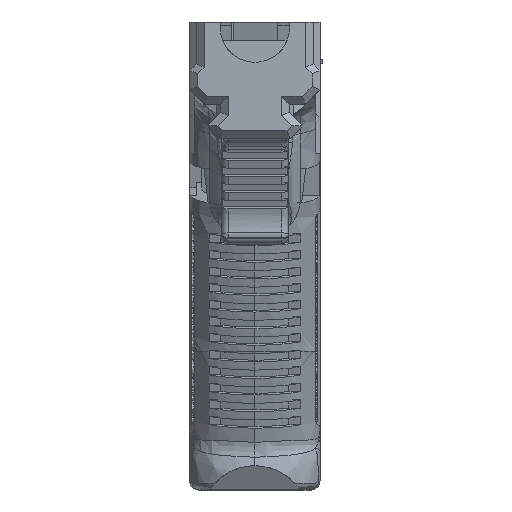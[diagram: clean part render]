
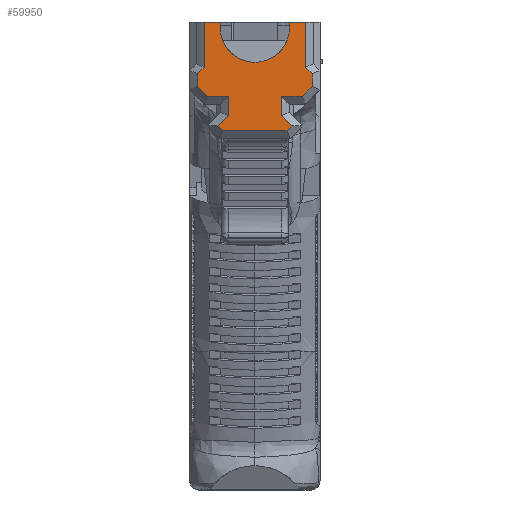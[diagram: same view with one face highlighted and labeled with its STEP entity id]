
A CAD part, left-side view. The second image highlights one B-rep face of the part: STEP entity #59950.
In plain terms, the highlighted planar face has unit normal (-1, 0, 0).
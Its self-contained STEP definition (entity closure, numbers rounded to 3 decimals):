
#7520=PLANE('',#61345);
#7623=LINE('',#68131,#11348);
#7689=LINE('',#70585,#11414);
#10973=LINE('',#139716,#14698);
#10977=LINE('',#139723,#14702);
#10980=LINE('',#139728,#14705);
#10982=LINE('',#139732,#14707);
#10984=LINE('',#139736,#14709);
#10986=LINE('',#139741,#14711);
#10997=LINE('',#139763,#14722);
#11000=LINE('',#139768,#14725);
#11002=LINE('',#139773,#14727);
#11014=LINE('',#139798,#14739);
#11016=LINE('',#139802,#14741);
#11018=LINE('',#139806,#14743);
#11020=LINE('',#139810,#14745);
#11022=LINE('',#139814,#14747);
#11025=LINE('',#139819,#14750);
#11239=LINE('',#142619,#14964);
#11241=LINE('',#142623,#14966);
#11242=LINE('',#142624,#14967);
#11243=LINE('',#142625,#14968);
#11348=VECTOR('',#61560,10.);
#11414=VECTOR('',#61656,10.);
#14698=VECTOR('',#67150,10.);
#14702=VECTOR('',#67156,10.);
#14705=VECTOR('',#67161,10.);
#14707=VECTOR('',#67165,10.);
#14709=VECTOR('',#67169,10.);
#14711=VECTOR('',#67173,10.);
#14722=VECTOR('',#67196,10.);
#14725=VECTOR('',#67201,10.);
#14727=VECTOR('',#67205,10.);
#14739=VECTOR('',#67229,10.);
#14741=VECTOR('',#67233,10.);
#14743=VECTOR('',#67237,10.);
#14745=VECTOR('',#67241,10.);
#14747=VECTOR('',#67245,10.);
#14750=VECTOR('',#67250,10.);
#14964=VECTOR('',#67768,10.);
#14966=VECTOR('',#67774,10.);
#14967=VECTOR('',#67775,10.);
#14968=VECTOR('',#67776,10.);
#18471=FACE_OUTER_BOUND('',#22299,.T.);
#22299=EDGE_LOOP('',(#56180,#56181,#56182,#56183,#56184,#56185,#56186,#56187,
#56188,#56189,#56190,#56191,#56192,#56193,#56194,#56195,#56196,#56197,#56198,
#56199,#56200,#56201));
#22546=CIRCLE('',#61247,7.765);
#23861=VERTEX_POINT('',#68128);
#23862=VERTEX_POINT('',#68130);
#24009=VERTEX_POINT('',#70582);
#24010=VERTEX_POINT('',#70584);
#29482=VERTEX_POINT('',#139713);
#29483=VERTEX_POINT('',#139715);
#29485=VERTEX_POINT('',#139721);
#29486=VERTEX_POINT('',#139726);
#29487=VERTEX_POINT('',#139730);
#29488=VERTEX_POINT('',#139734);
#29489=VERTEX_POINT('',#139738);
#29495=VERTEX_POINT('',#139762);
#29496=VERTEX_POINT('',#139766);
#29497=VERTEX_POINT('',#139770);
#29505=VERTEX_POINT('',#139797);
#29506=VERTEX_POINT('',#139801);
#29507=VERTEX_POINT('',#139805);
#29508=VERTEX_POINT('',#139809);
#29509=VERTEX_POINT('',#139813);
#29510=VERTEX_POINT('',#139818);
#29555=VERTEX_POINT('',#141368);
#29556=VERTEX_POINT('',#141370);
#29803=EDGE_CURVE('',#23862,#23861,#7623,.T.);
#29962=EDGE_CURVE('',#24010,#24009,#7689,.T.);
#38209=EDGE_CURVE('',#29482,#29483,#10973,.T.);
#38213=EDGE_CURVE('',#29485,#29482,#10977,.T.);
#38216=EDGE_CURVE('',#29486,#29485,#10980,.T.);
#38218=EDGE_CURVE('',#29487,#29486,#10982,.T.);
#38220=EDGE_CURVE('',#29488,#29487,#10984,.T.);
#38222=EDGE_CURVE('',#29489,#29488,#10986,.T.);
#38233=EDGE_CURVE('',#29495,#29489,#10997,.T.);
#38236=EDGE_CURVE('',#29496,#29495,#11000,.T.);
#38238=EDGE_CURVE('',#29497,#29496,#11002,.T.);
#38250=EDGE_CURVE('',#29505,#29497,#11014,.T.);
#38252=EDGE_CURVE('',#29506,#29505,#11016,.T.);
#38254=EDGE_CURVE('',#29507,#29506,#11018,.T.);
#38256=EDGE_CURVE('',#29508,#29507,#11020,.T.);
#38258=EDGE_CURVE('',#29509,#29508,#11022,.T.);
#38261=EDGE_CURVE('',#29510,#29509,#11025,.T.);
#38364=EDGE_CURVE('',#29556,#29555,#22546,.T.);
#38606=EDGE_CURVE('',#29483,#24009,#11239,.T.);
#38608=EDGE_CURVE('',#23861,#29556,#11241,.T.);
#38609=EDGE_CURVE('',#29555,#24010,#11242,.T.);
#38610=EDGE_CURVE('',#23862,#29510,#11243,.T.);
#56180=ORIENTED_EDGE('',*,*,#29803,.T.);
#56181=ORIENTED_EDGE('',*,*,#38608,.T.);
#56182=ORIENTED_EDGE('',*,*,#38364,.T.);
#56183=ORIENTED_EDGE('',*,*,#38609,.T.);
#56184=ORIENTED_EDGE('',*,*,#29962,.T.);
#56185=ORIENTED_EDGE('',*,*,#38606,.F.);
#56186=ORIENTED_EDGE('',*,*,#38209,.F.);
#56187=ORIENTED_EDGE('',*,*,#38213,.F.);
#56188=ORIENTED_EDGE('',*,*,#38216,.F.);
#56189=ORIENTED_EDGE('',*,*,#38218,.F.);
#56190=ORIENTED_EDGE('',*,*,#38220,.F.);
#56191=ORIENTED_EDGE('',*,*,#38222,.F.);
#56192=ORIENTED_EDGE('',*,*,#38233,.F.);
#56193=ORIENTED_EDGE('',*,*,#38236,.F.);
#56194=ORIENTED_EDGE('',*,*,#38238,.F.);
#56195=ORIENTED_EDGE('',*,*,#38250,.F.);
#56196=ORIENTED_EDGE('',*,*,#38252,.F.);
#56197=ORIENTED_EDGE('',*,*,#38254,.F.);
#56198=ORIENTED_EDGE('',*,*,#38256,.F.);
#56199=ORIENTED_EDGE('',*,*,#38258,.F.);
#56200=ORIENTED_EDGE('',*,*,#38261,.F.);
#56201=ORIENTED_EDGE('',*,*,#38610,.F.);
#59950=ADVANCED_FACE('',(#18471),#7520,.F.);
#61247=AXIS2_PLACEMENT_3D('',#141371,#67410,#67411);
#61345=AXIS2_PLACEMENT_3D('',#142622,#67772,#67773);
#61560=DIRECTION('',(0.,1.,0.));
#61656=DIRECTION('',(0.,1.,0.));
#67150=DIRECTION('',(0.,-0.707,0.707));
#67156=DIRECTION('',(0.,0.,1.));
#67161=DIRECTION('',(0.,0.707,0.707));
#67165=DIRECTION('',(0.,1.,0.));
#67169=DIRECTION('',(0.,0.,1.));
#67173=DIRECTION('',(0.,-0.707,0.707));
#67196=DIRECTION('',(0.,0.707,0.707));
#67201=DIRECTION('',(0.,1.,0.));
#67205=DIRECTION('',(0.,0.707,-0.707));
#67229=DIRECTION('',(0.,-0.707,-0.707));
#67233=DIRECTION('',(0.,0.,-1.));
#67237=DIRECTION('',(0.,1.,0.));
#67241=DIRECTION('',(0.,0.707,-0.707));
#67245=DIRECTION('',(0.,0.,-1.));
#67250=DIRECTION('',(0.,-0.707,-0.707));
#67410=DIRECTION('center_axis',(1.,0.,0.));
#67411=DIRECTION('ref_axis',(0.,0.,
-1.));
#67768=DIRECTION('',(0.,0.,1.));
#67772=DIRECTION('center_axis',(1.,0.,0.));
#67773=DIRECTION('ref_axis',(0.,0.,
1.));
#67774=DIRECTION('',(0.,0.,-1.));
#67775=DIRECTION('',(0.,0.,1.));
#67776=DIRECTION('',(0.,0.,-1.));
#68128=CARTESIAN_POINT('',(107.368,-102.914,-24.061));
#68130=CARTESIAN_POINT('',(107.368,-106.516,-24.061));
#68131=CARTESIAN_POINT('',(107.368,-106.726,-24.061));
#70582=CARTESIAN_POINT('',(107.368,-83.784,-24.061));
#70584=CARTESIAN_POINT('',(107.368,-87.386,-24.061));
#70585=CARTESIAN_POINT('',(107.368,-106.726,-24.061));
#139713=CARTESIAN_POINT('',(107.368,-82.284,-35.672));
#139715=CARTESIAN_POINT('',(107.368,-83.784,-34.172));
#139716=CARTESIAN_POINT('',(107.368,-83.976,-33.98));
#139721=CARTESIAN_POINT('',(107.368,-82.284,-38.526));
#139723=CARTESIAN_POINT('',(107.368,-82.284,-37.063));
#139726=CARTESIAN_POINT('',(107.368,-84.509,-40.75));
#139728=CARTESIAN_POINT('',(107.368,-91.325,-47.567));
#139730=CARTESIAN_POINT('',(107.368,-89.214,-40.75));
#139732=CARTESIAN_POINT('',(107.368,-99.114,-40.75));
#139734=CARTESIAN_POINT('',(107.368,-89.214,-45.067));
#139736=CARTESIAN_POINT('',(107.368,-89.214,-47.257));
#139738=CARTESIAN_POINT('',(107.368,-86.904,-47.377));
#139741=CARTESIAN_POINT('',(107.368,-89.763,-44.518));
#139762=CARTESIAN_POINT('',(107.368,-87.948,-48.421));
#139763=CARTESIAN_POINT('',(107.368,-91.713,-52.186));
#139766=CARTESIAN_POINT('',(107.368,-102.352,-48.421));
#139768=CARTESIAN_POINT('',(107.368,-95.,-48.421));
#139770=CARTESIAN_POINT('',(107.368,-103.396,-47.377));
#139773=CARTESIAN_POINT('',(107.368,-102.551,-48.223));
#139797=CARTESIAN_POINT('',(107.368,-101.086,-45.067));
#139798=CARTESIAN_POINT('',(107.368,-104.5,-48.481));
#139801=CARTESIAN_POINT('',(107.368,-101.086,-40.75));
#139802=CARTESIAN_POINT('',(107.368,-101.086,-47.257));
#139805=CARTESIAN_POINT('',(107.368,-105.791,-40.75));
#139806=CARTESIAN_POINT('',(107.368,-99.114,-40.75));
#139809=CARTESIAN_POINT('',(107.368,-108.016,-38.526));
#139810=CARTESIAN_POINT('',(107.368,-102.939,-43.603));
#139813=CARTESIAN_POINT('',(107.368,-108.016,-35.672));
#139814=CARTESIAN_POINT('',(107.368,-108.016,-37.063));
#139818=CARTESIAN_POINT('',(107.368,-106.516,-34.172));
#139819=CARTESIAN_POINT('',(107.368,-110.287,-37.943));
#141368=CARTESIAN_POINT('',(107.368,-87.386,-25.477));
#141370=CARTESIAN_POINT('',(107.368,-102.914,-25.477));
#141371=CARTESIAN_POINT('Origin',(107.368,-95.15,-25.35));
#142619=CARTESIAN_POINT('',(107.368,-83.784,-36.809));
#142622=CARTESIAN_POINT('Origin',(107.368,-103.077,-50.171));
#142623=CARTESIAN_POINT('',(107.368,-102.914,-32.455));
#142624=CARTESIAN_POINT('',(107.368,-87.386,-32.455));
#142625=CARTESIAN_POINT('',(107.368,-106.516,-36.809));
